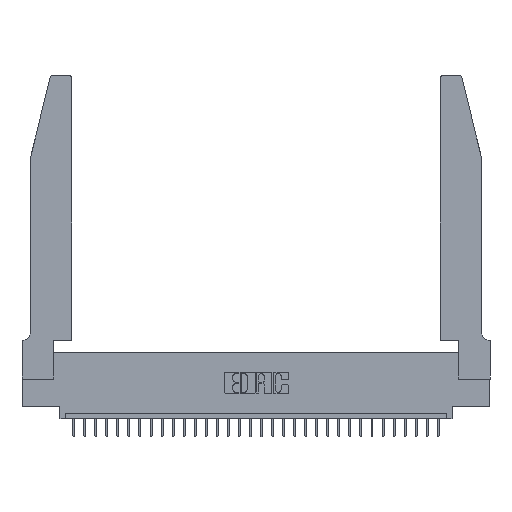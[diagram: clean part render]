
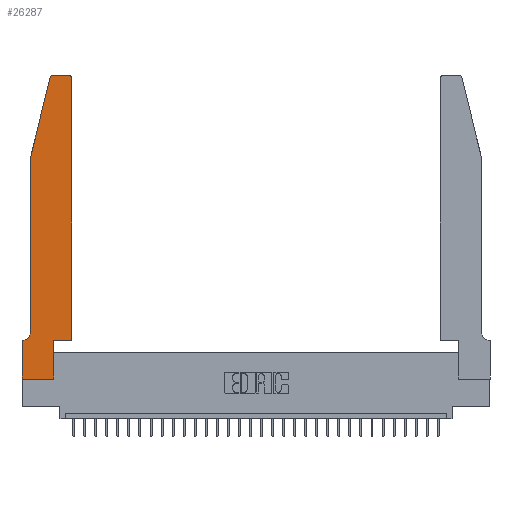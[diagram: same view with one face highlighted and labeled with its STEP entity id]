
A CAD part, top view. The second image highlights one B-rep face of the part: STEP entity #26287.
In plain terms, the highlighted planar face has unit normal (0, 0, 1).
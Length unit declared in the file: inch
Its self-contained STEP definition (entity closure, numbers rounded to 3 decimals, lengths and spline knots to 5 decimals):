
#409 = CARTESIAN_POINT ( 'NONE',  ( 0.0055, 0.35, 0.37 ) ) ;
#446 = DIRECTION ( 'NONE',  ( 0., -1., 0. ) ) ;
#1140 = ORIENTED_EDGE ( 'NONE', *, *, #17375, .T. ) ;
#1277 = CARTESIAN_POINT ( 'NONE',  ( 0., 0.35, 0.37 ) ) ;
#1620 = CARTESIAN_POINT ( 'NONE',  ( 0.4505, 0.35, 0.37 ) ) ;
#2057 = VECTOR ( 'NONE', #4774, 39.37008 ) ;
#2256 = VERTEX_POINT ( 'NONE', #28463 ) ;
#2407 = LINE ( 'NONE', #7115, #2057 ) ;
#2438 = LINE ( 'NONE', #1620, #15020 ) ;
#2459 = VERTEX_POINT ( 'NONE', #409 ) ;
#2939 = LINE ( 'NONE', #10331, #25947 ) ;
#3446 = CARTESIAN_POINT ( 'NONE',  ( 0., 0.35, 0.37 ) ) ;
#3622 = AXIS2_PLACEMENT_3D ( 'NONE', #6524, #8539, #7708 ) ;
#3631 = CARTESIAN_POINT ( 'NONE',  ( 0.0755, 0.35, 0.37 ) ) ;
#3737 = VECTOR ( 'NONE', #15611, 39.37008 ) ;
#3832 = LINE ( 'NONE', #30403, #22582 ) ;
#3921 = DIRECTION ( 'NONE',  ( 1., 0., 0. ) ) ;
#3966 = CARTESIAN_POINT ( 'NONE',  ( 0.0755, 2., 0.37 ) ) ;
#4774 = DIRECTION ( 'NONE',  ( 1., 0., 0. ) ) ;
#5424 = CARTESIAN_POINT ( 'NONE',  ( 0., 0., 0.37 ) ) ;
#5480 = CARTESIAN_POINT ( 'NONE',  ( 0.284, 2.75, 0.37 ) ) ;
#5714 = EDGE_CURVE ( 'NONE', #16507, #6336, #21751, .T. ) ;
#5764 = DIRECTION ( 'NONE',  ( 1., 0., 0. ) ) ;
#5803 = CARTESIAN_POINT ( 'NONE',  ( 0.25487, 2.72718, 0.37 ) ) ;
#6336 = VERTEX_POINT ( 'NONE', #9265 ) ;
#6352 = ORIENTED_EDGE ( 'NONE', *, *, #29536, .T. ) ;
#6361 = EDGE_CURVE ( 'NONE', #15708, #12084, #16036, .T. ) ;
#6524 = CARTESIAN_POINT ( 'NONE',  ( 0.0055, 0.42, 0.37 ) ) ;
#6719 = ORIENTED_EDGE ( 'NONE', *, *, #10789, .T. ) ;
#6787 = CARTESIAN_POINT ( 'NONE',  ( 0.4505, 0.35, 0.37 ) ) ;
#7115 = CARTESIAN_POINT ( 'NONE',  ( 0.4505, 0.35, 0.37 ) ) ;
#7708 = DIRECTION ( 'NONE',  ( -1., 0., 0. ) ) ;
#8539 = DIRECTION ( 'NONE',  ( 0., 0., -1. ) ) ;
#8698 = LINE ( 'NONE', #3631, #3737 ) ;
#9242 = AXIS2_PLACEMENT_3D ( 'NONE', #31621, #21385, #23938 ) ;
#9265 = CARTESIAN_POINT ( 'NONE',  ( 0.2865, 0.35, 0.37 ) ) ;
#9337 = EDGE_CURVE ( 'NONE', #12084, #13593, #17707, .T. ) ;
#9502 = CARTESIAN_POINT ( 'NONE',  ( 0.4505, 2.72, 0.37 ) ) ;
#10116 = DIRECTION ( 'NONE',  ( 1., 0., 0. ) ) ;
#10331 = CARTESIAN_POINT ( 'NONE',  ( 0., 0., 0.37 ) ) ;
#10541 = ORIENTED_EDGE ( 'NONE', *, *, #5714, .T. ) ;
#10789 = EDGE_CURVE ( 'NONE', #10879, #2256, #16896, .T. ) ;
#10879 = VERTEX_POINT ( 'NONE', #3446 ) ;
#11003 = CIRCLE ( 'NONE', #19708, 0.03 ) ;
#12084 = VERTEX_POINT ( 'NONE', #5803 ) ;
#12122 = EDGE_CURVE ( 'NONE', #16771, #15708, #3832, .T. ) ;
#12124 = AXIS2_PLACEMENT_3D ( 'NONE', #1277, #13662, #3921 ) ;
#12420 = CARTESIAN_POINT ( 'NONE',  ( 0.0755, 0.42, 0.37 ) ) ;
#12523 = CIRCLE ( 'NONE', #3622, 0.07 ) ;
#13202 = EDGE_CURVE ( 'NONE', #15517, #2459, #12523, .T. ) ;
#13593 = VERTEX_POINT ( 'NONE', #20557 ) ;
#13662 = DIRECTION ( 'NONE',  ( 0., 0., 1. ) ) ;
#13738 = ORIENTED_EDGE ( 'NONE', *, *, #9337, .T. ) ;
#13813 = CARTESIAN_POINT ( 'NONE',  ( 0.2865, 0., 0.37 ) ) ;
#15020 = VECTOR ( 'NONE', #16052, 39.37008 ) ;
#15233 = VECTOR ( 'NONE', #19281, 39.37008 ) ;
#15517 = VERTEX_POINT ( 'NONE', #12420 ) ;
#15611 = DIRECTION ( 'NONE',  ( -1., 0., 0. ) ) ;
#15708 = VERTEX_POINT ( 'NONE', #5480 ) ;
#15924 = FACE_OUTER_BOUND ( 'NONE', #17141, .T. ) ;
#15945 = CARTESIAN_POINT ( 'NONE',  ( 0.4205, 2.72, 0.37 ) ) ;
#16036 = CIRCLE ( 'NONE', #9242, 0.03 ) ;
#16052 = DIRECTION ( 'NONE',  ( 0., 1., 0. ) ) ;
#16507 = VERTEX_POINT ( 'NONE', #13813 ) ;
#16771 = VERTEX_POINT ( 'NONE', #31127 ) ;
#16896 = LINE ( 'NONE', #5424, #17629 ) ;
#17141 = EDGE_LOOP ( 'NONE', ( #26466, #24150, #13738, #6352, #29614, #1140, #6719, #22365, #10541, #26929, #24620, #19476 ) ) ;
#17317 = EDGE_CURVE ( 'NONE', #22546, #16771, #11003, .T. ) ;
#17375 = EDGE_CURVE ( 'NONE', #2459, #10879, #8698, .T. ) ;
#17629 = VECTOR ( 'NONE', #446, 39.37008 ) ;
#17707 = LINE ( 'NONE', #3966, #31490 ) ;
#19281 = DIRECTION ( 'NONE',  ( 0., 1., 0. ) ) ;
#19476 = ORIENTED_EDGE ( 'NONE', *, *, #17317, .T. ) ;
#19708 = AXIS2_PLACEMENT_3D ( 'NONE', #15945, #20868, #5764 ) ;
#20048 = EDGE_CURVE ( 'NONE', #6336, #21463, #2407, .T. ) ;
#20557 = CARTESIAN_POINT ( 'NONE',  ( 0.0755, 2., 0.37 ) ) ;
#20868 = DIRECTION ( 'NONE',  ( 0., 0., 1. ) ) ;
#21108 = DIRECTION ( 'NONE',  ( -0.239, -0.971, 0. ) ) ;
#21327 = CARTESIAN_POINT ( 'NONE',  ( 0.0755, 2., 0.37 ) ) ;
#21385 = DIRECTION ( 'NONE',  ( 0., 0., 1. ) ) ;
#21463 = VERTEX_POINT ( 'NONE', #6787 ) ;
#21751 = LINE ( 'NONE', #31450, #15233 ) ;
#21980 = LINE ( 'NONE', #21327, #30796 ) ;
#22365 = ORIENTED_EDGE ( 'NONE', *, *, #25568, .T. ) ;
#22546 = VERTEX_POINT ( 'NONE', #9502 ) ;
#22582 = VECTOR ( 'NONE', #22919, 39.37008 ) ;
#22919 = DIRECTION ( 'NONE',  ( -1., 0., 0. ) ) ;
#23938 = DIRECTION ( 'NONE',  ( 1., 0., 0. ) ) ;
#24150 = ORIENTED_EDGE ( 'NONE', *, *, #6361, .T. ) ;
#24620 = ORIENTED_EDGE ( 'NONE', *, *, #30000, .T. ) ;
#25568 = EDGE_CURVE ( 'NONE', #2256, #16507, #2939, .T. ) ;
#25947 = VECTOR ( 'NONE', #10116, 39.37008 ) ;
#26287 = ADVANCED_FACE ( 'NONE', ( #15924 ), #30446, .T. ) ;
#26466 = ORIENTED_EDGE ( 'NONE', *, *, #12122, .T. ) ;
#26483 = DIRECTION ( 'NONE',  ( 0., -1., 0. ) ) ;
#26929 = ORIENTED_EDGE ( 'NONE', *, *, #20048, .T. ) ;
#28463 = CARTESIAN_POINT ( 'NONE',  ( 0., 0., 0.37 ) ) ;
#29536 = EDGE_CURVE ( 'NONE', #13593, #15517, #21980, .T. ) ;
#29614 = ORIENTED_EDGE ( 'NONE', *, *, #13202, .T. ) ;
#30000 = EDGE_CURVE ( 'NONE', #21463, #22546, #2438, .T. ) ;
#30403 = CARTESIAN_POINT ( 'NONE',  ( 0.2605, 2.75, 0.37 ) ) ;
#30446 = PLANE ( 'NONE',  #12124 ) ;
#30796 = VECTOR ( 'NONE', #26483, 39.37008 ) ;
#31127 = CARTESIAN_POINT ( 'NONE',  ( 0.4205, 2.75, 0.37 ) ) ;
#31450 = CARTESIAN_POINT ( 'NONE',  ( 0.2865, 0.35, 0.37 ) ) ;
#31490 = VECTOR ( 'NONE', #21108, 39.37008 ) ;
#31621 = CARTESIAN_POINT ( 'NONE',  ( 0.284, 2.72, 0.37 ) ) ;
